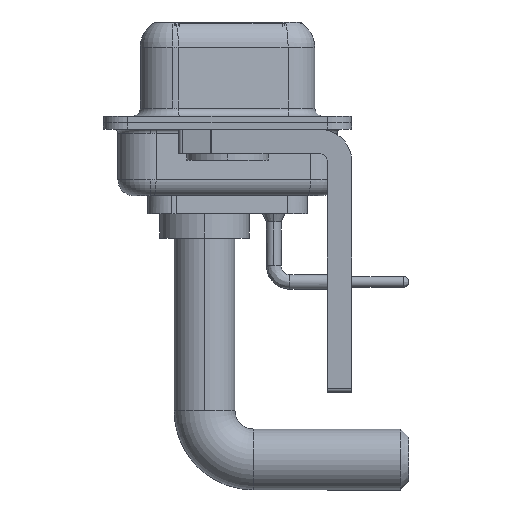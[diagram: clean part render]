
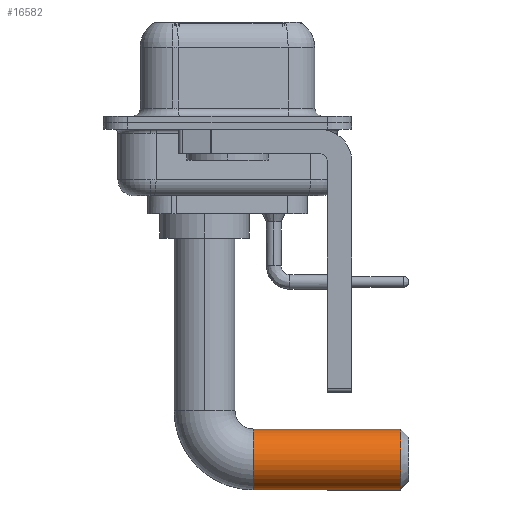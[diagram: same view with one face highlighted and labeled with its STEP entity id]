
A CAD part, left-side view. The second image highlights one B-rep face of the part: STEP entity #16582.
In plain terms, the highlighted cylindrical face has radius 1.875 mm (diameter 3.75 mm), a partial arc.
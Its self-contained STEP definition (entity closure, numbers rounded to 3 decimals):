
#340 = AXIS2_PLACEMENT_3D ( 'NONE', #16181, #3989, #14738 ) ;
#1345 = FACE_OUTER_BOUND ( 'NONE', #8107, .T. ) ;
#1378 = DIRECTION ( 'NONE',  ( 0., -1., 0. ) ) ;
#3000 = CARTESIAN_POINT ( 'NONE',  ( 0., -3., -15.505 ) ) ;
#3885 = ORIENTED_EDGE ( 'NONE', *, *, #4560, .F. ) ;
#3989 = DIRECTION ( 'NONE',  ( 0., -1., 0. ) ) ;
#4560 = EDGE_CURVE ( 'NONE', #6155, #17006, #16623, .T. ) ;
#5872 = VERTEX_POINT ( 'NONE', #3000 ) ;
#6065 = CARTESIAN_POINT ( 'NONE',  ( 0., -3., -11.755 ) ) ;
#6155 = VERTEX_POINT ( 'NONE', #6065 ) ;
#6474 = CYLINDRICAL_SURFACE ( 'NONE', #6913, 1.875 ) ;
#6913 = AXIS2_PLACEMENT_3D ( 'NONE', #13153, #16589, #8144 ) ;
#8107 = EDGE_LOOP ( 'NONE', ( #3885, #18994, #15756, #20904 ) ) ;
#8144 = DIRECTION ( 'NONE',  ( 0., 0., -1. ) ) ;
#8941 = VERTEX_POINT ( 'NONE', #19450 ) ;
#10811 = LINE ( 'NONE', #20901, #11831 ) ;
#10941 = EDGE_CURVE ( 'NONE', #6155, #5872, #16673, .T. ) ;
#11831 = VECTOR ( 'NONE', #21007, 1000. ) ;
#12970 = DIRECTION ( 'NONE',  ( 0., 0., -1. ) ) ;
#13153 = CARTESIAN_POINT ( 'NONE',  ( 0., -3., -13.63 ) ) ;
#13184 = CARTESIAN_POINT ( 'NONE',  ( 0., -3., -11.755 ) ) ;
#13772 = CARTESIAN_POINT ( 'NONE',  ( 0., -12.07, -11.755 ) ) ;
#14205 = VECTOR ( 'NONE', #1378, 1000. ) ;
#14455 = CIRCLE ( 'NONE', #15863, 1.875 ) ;
#14738 = DIRECTION ( 'NONE',  ( -1., 0., 0. ) ) ;
#15468 = EDGE_CURVE ( 'NONE', #5872, #8941, #10811, .T. ) ;
#15756 = ORIENTED_EDGE ( 'NONE', *, *, #15468, .T. ) ;
#15863 = AXIS2_PLACEMENT_3D ( 'NONE', #21408, #17957, #12970 ) ;
#16181 = CARTESIAN_POINT ( 'NONE',  ( 0., -3., -13.63 ) ) ;
#16582 = ADVANCED_FACE ( 'NONE', ( #1345 ), #6474, .T. ) ;
#16589 = DIRECTION ( 'NONE',  ( 0., -1., 0. ) ) ;
#16623 = LINE ( 'NONE', #13184, #14205 ) ;
#16673 = CIRCLE ( 'NONE', #340, 1.875 ) ;
#17006 = VERTEX_POINT ( 'NONE', #13772 ) ;
#17957 = DIRECTION ( 'NONE',  ( 0., 1., 0. ) ) ;
#18994 = ORIENTED_EDGE ( 'NONE', *, *, #10941, .T. ) ;
#19450 = CARTESIAN_POINT ( 'NONE',  ( 0., -12.07, -15.505 ) ) ;
#20432 = EDGE_CURVE ( 'NONE', #8941, #17006, #14455, .T. ) ;
#20901 = CARTESIAN_POINT ( 'NONE',  ( 0., -3., -15.505 ) ) ;
#20904 = ORIENTED_EDGE ( 'NONE', *, *, #20432, .T. ) ;
#21007 = DIRECTION ( 'NONE',  ( 0., -1., 0. ) ) ;
#21408 = CARTESIAN_POINT ( 'NONE',  ( 0., -12.07, -13.63 ) ) ;
